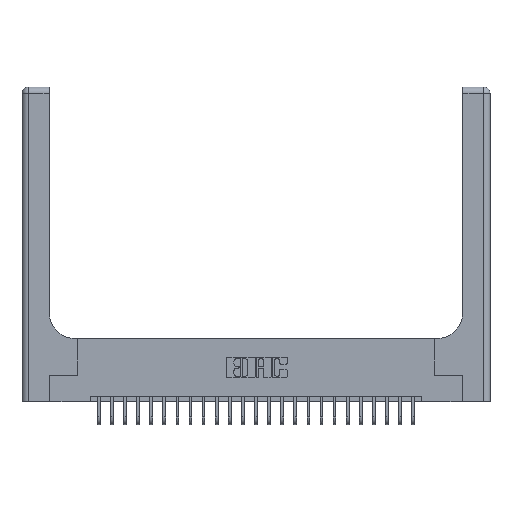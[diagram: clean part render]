
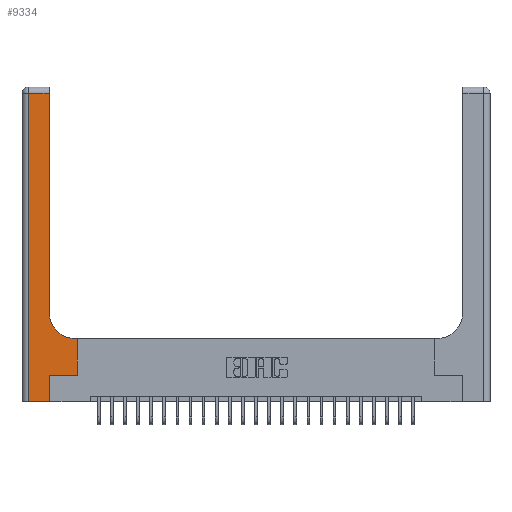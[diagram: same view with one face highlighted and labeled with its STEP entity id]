
A CAD part, top view. The second image highlights one B-rep face of the part: STEP entity #9334.
In plain terms, the highlighted planar face has unit normal (0, 0, 1).
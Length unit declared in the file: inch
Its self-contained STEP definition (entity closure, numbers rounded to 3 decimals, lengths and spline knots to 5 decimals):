
#374 = EDGE_LOOP ( 'NONE', ( #14858, #12621, #6988, #25717, #9410, #22846, #6705, #20381, #15360 ) ) ;
#1008 = VECTOR ( 'NONE', #3885, 39.37008 ) ;
#1150 = VECTOR ( 'NONE', #20592, 39.37008 ) ;
#1163 = CARTESIAN_POINT ( 'NONE',  ( 0., 3., 0.37 ) ) ;
#1351 = LINE ( 'NONE', #17433, #8161 ) ;
#1584 = LINE ( 'NONE', #10011, #4129 ) ;
#1787 = CARTESIAN_POINT ( 'NONE',  ( 0.26, 3., 0.37 ) ) ;
#1908 = EDGE_CURVE ( 'NONE', #11134, #20736, #4166, .T. ) ;
#1920 = CARTESIAN_POINT ( 'NONE',  ( 0.06, 2.94, 0.37 ) ) ;
#2252 = EDGE_CURVE ( 'NONE', #3735, #17299, #17294, .T. ) ;
#2797 = CARTESIAN_POINT ( 'NONE',  ( 0., 2.94, 0.37 ) ) ;
#3261 = FACE_OUTER_BOUND ( 'NONE', #374, .T. ) ;
#3735 = VERTEX_POINT ( 'NONE', #24703 ) ;
#3885 = DIRECTION ( 'NONE',  ( 0., 1., 0. ) ) ;
#4129 = VECTOR ( 'NONE', #17660, 39.37008 ) ;
#4166 = LINE ( 'NONE', #22096, #6081 ) ;
#4357 = EDGE_CURVE ( 'NONE', #20736, #17391, #1584, .T. ) ;
#4515 = LINE ( 'NONE', #6221, #14447 ) ;
#4766 = LINE ( 'NONE', #2797, #1150 ) ;
#5042 = CARTESIAN_POINT ( 'NONE',  ( 0.265, 0.25, 0.37 ) ) ;
#6081 = VECTOR ( 'NONE', #21965, 39.37008 ) ;
#6221 = CARTESIAN_POINT ( 'NONE',  ( 0.06, 3., 0.37 ) ) ;
#6281 = CARTESIAN_POINT ( 'NONE',  ( 0.26, 2.94, 0.37 ) ) ;
#6705 = ORIENTED_EDGE ( 'NONE', *, *, #4357, .T. ) ;
#6988 = ORIENTED_EDGE ( 'NONE', *, *, #24180, .T. ) ;
#7854 = DIRECTION ( 'NONE',  ( -1., 0., 0. ) ) ;
#8161 = VECTOR ( 'NONE', #21266, 39.37008 ) ;
#8395 = CARTESIAN_POINT ( 'NONE',  ( 0.265, 0., 0.37 ) ) ;
#9042 = EDGE_CURVE ( 'NONE', #18811, #11134, #18312, .T. ) ;
#9153 = DIRECTION ( 'NONE',  ( 1., 0., 0. ) ) ;
#9334 = ADVANCED_FACE ( 'NONE', ( #3261 ), #11157, .F. ) ;
#9410 = ORIENTED_EDGE ( 'NONE', *, *, #9042, .T. ) ;
#9692 = DIRECTION ( 'NONE',  ( 0., 0., -1. ) ) ;
#10011 = CARTESIAN_POINT ( 'NONE',  ( 0.528, 0.25, 0.37 ) ) ;
#10923 = EDGE_CURVE ( 'NONE', #17299, #13858, #22208, .T. ) ;
#11134 = VERTEX_POINT ( 'NONE', #5042 ) ;
#11157 = PLANE ( 'NONE',  #16928 ) ;
#11249 = CARTESIAN_POINT ( 'NONE',  ( 0.51, 0.85, 0.37 ) ) ;
#11503 = DIRECTION ( 'NONE',  ( 0., 0., -1. ) ) ;
#12543 = DIRECTION ( 'NONE',  ( 0., -1., 0. ) ) ;
#12621 = ORIENTED_EDGE ( 'NONE', *, *, #16671, .T. ) ;
#12715 = CARTESIAN_POINT ( 'NONE',  ( 0.528, 0.25, 0.37 ) ) ;
#12741 = EDGE_CURVE ( 'NONE', #23725, #18811, #1351, .T. ) ;
#13115 = VECTOR ( 'NONE', #24248, 39.37008 ) ;
#13858 = VERTEX_POINT ( 'NONE', #6281 ) ;
#14447 = VECTOR ( 'NONE', #12543, 39.37008 ) ;
#14858 = ORIENTED_EDGE ( 'NONE', *, *, #10923, .T. ) ;
#15258 = EDGE_CURVE ( 'NONE', #17391, #3735, #18140, .T. ) ;
#15360 = ORIENTED_EDGE ( 'NONE', *, *, #2252, .T. ) ;
#15934 = CARTESIAN_POINT ( 'NONE',  ( 0.528, 0.6, 0.37 ) ) ;
#16671 = EDGE_CURVE ( 'NONE', #13858, #25496, #4766, .T. ) ;
#16928 = AXIS2_PLACEMENT_3D ( 'NONE', #1163, #9692, #25264 ) ;
#17294 = CIRCLE ( 'NONE', #18158, 0.25 ) ;
#17299 = VERTEX_POINT ( 'NONE', #17506 ) ;
#17391 = VERTEX_POINT ( 'NONE', #15934 ) ;
#17433 = CARTESIAN_POINT ( 'NONE',  ( 0., 0., 0.37 ) ) ;
#17506 = CARTESIAN_POINT ( 'NONE',  ( 0.26, 0.85, 0.37 ) ) ;
#17660 = DIRECTION ( 'NONE',  ( 0., 1., 0. ) ) ;
#18140 = LINE ( 'NONE', #25777, #22542 ) ;
#18158 = AXIS2_PLACEMENT_3D ( 'NONE', #11249, #11503, #9153 ) ;
#18312 = LINE ( 'NONE', #20037, #13115 ) ;
#18811 = VERTEX_POINT ( 'NONE', #8395 ) ;
#20037 = CARTESIAN_POINT ( 'NONE',  ( 0.265, 0., 0.37 ) ) ;
#20381 = ORIENTED_EDGE ( 'NONE', *, *, #15258, .T. ) ;
#20592 = DIRECTION ( 'NONE',  ( -1., 0., 0. ) ) ;
#20736 = VERTEX_POINT ( 'NONE', #12715 ) ;
#21266 = DIRECTION ( 'NONE',  ( 1., 0., 0. ) ) ;
#21965 = DIRECTION ( 'NONE',  ( 1., 0., 0. ) ) ;
#22096 = CARTESIAN_POINT ( 'NONE',  ( 0.265, 0.25, 0.37 ) ) ;
#22208 = LINE ( 'NONE', #1787, #1008 ) ;
#22542 = VECTOR ( 'NONE', #7854, 39.37008 ) ;
#22716 = CARTESIAN_POINT ( 'NONE',  ( 0.06, 0., 0.37 ) ) ;
#22846 = ORIENTED_EDGE ( 'NONE', *, *, #1908, .T. ) ;
#23725 = VERTEX_POINT ( 'NONE', #22716 ) ;
#24180 = EDGE_CURVE ( 'NONE', #25496, #23725, #4515, .T. ) ;
#24248 = DIRECTION ( 'NONE',  ( 0., 1., 0. ) ) ;
#24703 = CARTESIAN_POINT ( 'NONE',  ( 0.51, 0.6, 0.37 ) ) ;
#25264 = DIRECTION ( 'NONE',  ( -1., 0., 0. ) ) ;
#25496 = VERTEX_POINT ( 'NONE', #1920 ) ;
#25717 = ORIENTED_EDGE ( 'NONE', *, *, #12741, .T. ) ;
#25777 = CARTESIAN_POINT ( 'NONE',  ( 0.26, 0.6, 0.37 ) ) ;
